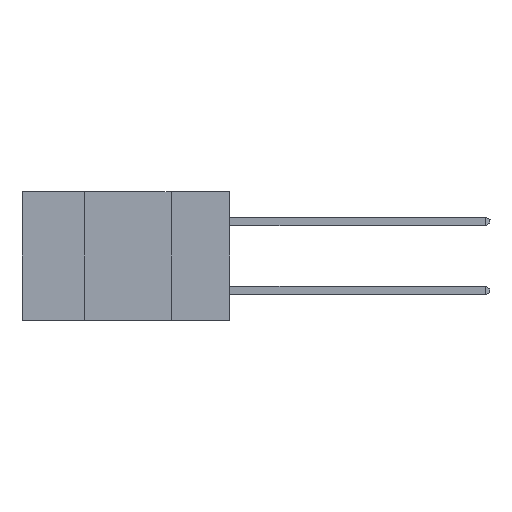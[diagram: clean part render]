
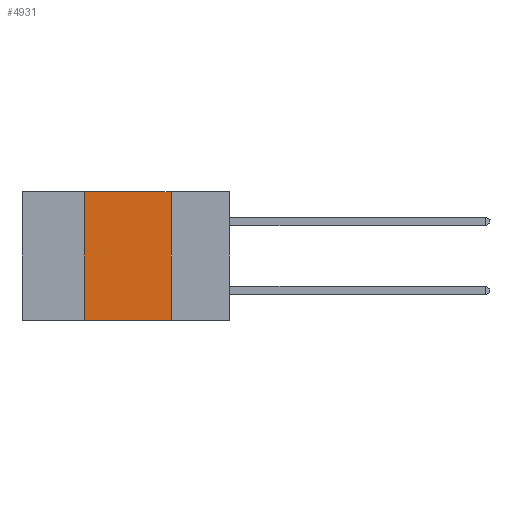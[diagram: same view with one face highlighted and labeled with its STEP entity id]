
A CAD part, left-side view. The second image highlights one B-rep face of the part: STEP entity #4931.
In plain terms, the highlighted planar face has unit normal (-1, 0, 0).
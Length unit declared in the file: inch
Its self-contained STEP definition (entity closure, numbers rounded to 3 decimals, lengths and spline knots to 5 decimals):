
#631 = LINE ( 'NONE', #8891, #12217 ) ;
#1285 = DIRECTION ( 'NONE',  ( 0., 0., 1. ) ) ;
#1632 = ORIENTED_EDGE ( 'NONE', *, *, #3405, .F. ) ;
#1746 = FACE_OUTER_BOUND ( 'NONE', #6401, .T. ) ;
#2199 = VERTEX_POINT ( 'NONE', #2777 ) ;
#2607 = EDGE_CURVE ( 'NONE', #13325, #9985, #2818, .T. ) ;
#2777 = CARTESIAN_POINT ( 'NONE',  ( 0., 0.17, -0.37 ) ) ;
#2818 = LINE ( 'NONE', #8017, #7659 ) ;
#3016 = CARTESIAN_POINT ( 'NONE',  ( 0., 0.42, 0. ) ) ;
#3103 = DIRECTION ( 'NONE',  ( 0., -1., 0. ) ) ;
#3273 = DIRECTION ( 'NONE',  ( 1., 0., 0. ) ) ;
#3405 = EDGE_CURVE ( 'NONE', #10021, #13325, #15621, .T. ) ;
#4037 = CARTESIAN_POINT ( 'NONE',  ( 0., 0.42, 0. ) ) ;
#4540 = VECTOR ( 'NONE', #1285, 39.37008 ) ;
#4587 = DIRECTION ( 'NONE',  ( 0., 0., -1. ) ) ;
#4931 = ADVANCED_FACE ( 'NONE', ( #1746 ), #11792, .F. ) ;
#5993 = DIRECTION ( 'NONE',  ( 0., 0., -1. ) ) ;
#6401 = EDGE_LOOP ( 'NONE', ( #13945, #13227, #1632, #8111 ) ) ;
#7659 = VECTOR ( 'NONE', #16541, 39.37008 ) ;
#7722 = VECTOR ( 'NONE', #3103, 39.37008 ) ;
#8017 = CARTESIAN_POINT ( 'NONE',  ( 0., 0.6, 0. ) ) ;
#8111 = ORIENTED_EDGE ( 'NONE', *, *, #12495, .T. ) ;
#8891 = CARTESIAN_POINT ( 'NONE',  ( 0., 0.17, 0. ) ) ;
#9985 = VERTEX_POINT ( 'NONE', #15326 ) ;
#10021 = VERTEX_POINT ( 'NONE', #16969 ) ;
#11792 = PLANE ( 'NONE',  #17816 ) ;
#11853 = EDGE_CURVE ( 'NONE', #9985, #2199, #631, .T. ) ;
#12217 = VECTOR ( 'NONE', #5993, 39.37008 ) ;
#12495 = EDGE_CURVE ( 'NONE', #10021, #2199, #15271, .T. ) ;
#13157 = CARTESIAN_POINT ( 'NONE',  ( 0., 0.6, 0. ) ) ;
#13227 = ORIENTED_EDGE ( 'NONE', *, *, #2607, .F. ) ;
#13325 = VERTEX_POINT ( 'NONE', #3016 ) ;
#13945 = ORIENTED_EDGE ( 'NONE', *, *, #11853, .F. ) ;
#15271 = LINE ( 'NONE', #17142, #7722 ) ;
#15326 = CARTESIAN_POINT ( 'NONE',  ( 0., 0.17, 0. ) ) ;
#15621 = LINE ( 'NONE', #4037, #4540 ) ;
#16541 = DIRECTION ( 'NONE',  ( 0., -1., 0. ) ) ;
#16969 = CARTESIAN_POINT ( 'NONE',  ( 0., 0.42, -0.37 ) ) ;
#17142 = CARTESIAN_POINT ( 'NONE',  ( 0., 0.6, -0.37 ) ) ;
#17816 = AXIS2_PLACEMENT_3D ( 'NONE', #13157, #3273, #4587 ) ;
